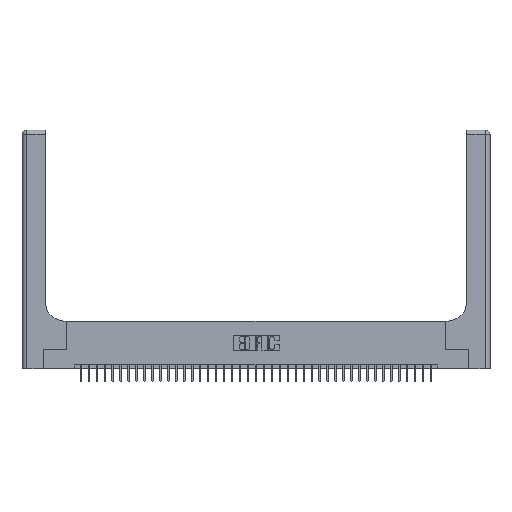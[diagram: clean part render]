
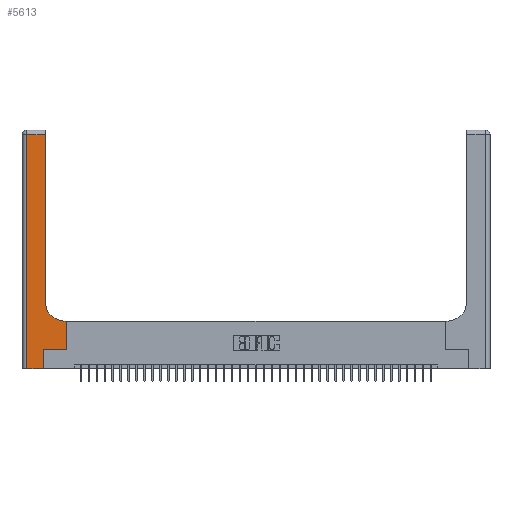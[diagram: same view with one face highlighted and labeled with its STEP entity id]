
A CAD part, top view. The second image highlights one B-rep face of the part: STEP entity #5613.
In plain terms, the highlighted planar face has unit normal (0, 0, 1).
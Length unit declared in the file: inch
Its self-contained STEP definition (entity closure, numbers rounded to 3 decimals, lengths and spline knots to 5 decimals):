
#130 = CARTESIAN_POINT ( 'NONE',  ( 0.06, 3., 0.37 ) ) ;
#830 = VECTOR ( 'NONE', #20768, 39.37008 ) ;
#1373 = CARTESIAN_POINT ( 'NONE',  ( 0.5415, 0.85, 0.37 ) ) ;
#3284 = DIRECTION ( 'NONE',  ( 0., -1., 0. ) ) ;
#3754 = CARTESIAN_POINT ( 'NONE',  ( 0.5585, 0.6, 0.37 ) ) ;
#3790 = VERTEX_POINT ( 'NONE', #15621 ) ;
#4520 = DIRECTION ( 'NONE',  ( 1., 0., 0. ) ) ;
#4714 = LINE ( 'NONE', #38202, #35749 ) ;
#4879 = LINE ( 'NONE', #14296, #12200 ) ;
#4936 = DIRECTION ( 'NONE',  ( 0., 1., 0. ) ) ;
#4947 = VECTOR ( 'NONE', #11902, 39.37008 ) ;
#5030 = ORIENTED_EDGE ( 'NONE', *, *, #28999, .T. ) ;
#5613 = ADVANCED_FACE ( 'NONE', ( #12121 ), #33946, .F. ) ;
#6167 = DIRECTION ( 'NONE',  ( -1., 0., 0. ) ) ;
#6580 = VERTEX_POINT ( 'NONE', #35375 ) ;
#6622 = DIRECTION ( 'NONE',  ( 1., 0., 0. ) ) ;
#7062 = EDGE_CURVE ( 'NONE', #3790, #25156, #9646, .T. ) ;
#7198 = LINE ( 'NONE', #130, #15441 ) ;
#9646 = LINE ( 'NONE', #15824, #23162 ) ;
#10445 = EDGE_CURVE ( 'NONE', #6580, #27169, #28688, .T. ) ;
#11052 = CARTESIAN_POINT ( 'NONE',  ( 0., 2.94, 0.37 ) ) ;
#11204 = ORIENTED_EDGE ( 'NONE', *, *, #7062, .T. ) ;
#11902 = DIRECTION ( 'NONE',  ( 0., 1., 0. ) ) ;
#12121 = FACE_OUTER_BOUND ( 'NONE', #28138, .T. ) ;
#12200 = VECTOR ( 'NONE', #4936, 39.37008 ) ;
#12298 = CARTESIAN_POINT ( 'NONE',  ( 0., 3., 0.37 ) ) ;
#13057 = DIRECTION ( 'NONE',  ( -1., 0., 0. ) ) ;
#13212 = LINE ( 'NONE', #14846, #4947 ) ;
#14142 = DIRECTION ( 'NONE',  ( -1., 0., 0. ) ) ;
#14296 = CARTESIAN_POINT ( 'NONE',  ( 0.5585, 0.25, 0.37 ) ) ;
#14688 = LINE ( 'NONE', #28485, #38421 ) ;
#14846 = CARTESIAN_POINT ( 'NONE',  ( 0.2915, 3., 0.37 ) ) ;
#15441 = VECTOR ( 'NONE', #3284, 39.37008 ) ;
#15621 = CARTESIAN_POINT ( 'NONE',  ( 0.06, 0., 0.37 ) ) ;
#15824 = CARTESIAN_POINT ( 'NONE',  ( 0., 0., 0.37 ) ) ;
#16118 = CARTESIAN_POINT ( 'NONE',  ( 0.5415, 0.6, 0.37 ) ) ;
#16372 = EDGE_CURVE ( 'NONE', #21794, #37944, #4879, .T. ) ;
#16645 = VERTEX_POINT ( 'NONE', #27847 ) ;
#16713 = VERTEX_POINT ( 'NONE', #21866 ) ;
#17464 = CIRCLE ( 'NONE', #35033, 0.25 ) ;
#17623 = CARTESIAN_POINT ( 'NONE',  ( 0.269, 0.25, 0.37 ) ) ;
#17897 = ORIENTED_EDGE ( 'NONE', *, *, #31254, .T. ) ;
#18410 = AXIS2_PLACEMENT_3D ( 'NONE', #12298, #24723, #6167 ) ;
#18676 = VERTEX_POINT ( 'NONE', #16118 ) ;
#19835 = EDGE_CURVE ( 'NONE', #16713, #6580, #13212, .T. ) ;
#20459 = VECTOR ( 'NONE', #14142, 39.37008 ) ;
#20768 = DIRECTION ( 'NONE',  ( 1., 0., 0. ) ) ;
#20869 = ORIENTED_EDGE ( 'NONE', *, *, #10445, .T. ) ;
#21530 = CARTESIAN_POINT ( 'NONE',  ( 0.5585, 0.25, 0.37 ) ) ;
#21794 = VERTEX_POINT ( 'NONE', #21530 ) ;
#21866 = CARTESIAN_POINT ( 'NONE',  ( 0.2915, 0.85, 0.37 ) ) ;
#22688 = CARTESIAN_POINT ( 'NONE',  ( 0.06, 2.94, 0.37 ) ) ;
#22755 = DIRECTION ( 'NONE',  ( 0., 1., 0. ) ) ;
#23087 = DIRECTION ( 'NONE',  ( 0., 0., -1. ) ) ;
#23162 = VECTOR ( 'NONE', #6622, 39.37008 ) ;
#24457 = CARTESIAN_POINT ( 'NONE',  ( 0.269, 0., 0.37 ) ) ;
#24723 = DIRECTION ( 'NONE',  ( 0., 0., -1. ) ) ;
#25156 = VERTEX_POINT ( 'NONE', #24457 ) ;
#25208 = ORIENTED_EDGE ( 'NONE', *, *, #19835, .T. ) ;
#25587 = LINE ( 'NONE', #17623, #830 ) ;
#27169 = VERTEX_POINT ( 'NONE', #22688 ) ;
#27688 = EDGE_CURVE ( 'NONE', #37944, #18676, #14688, .T. ) ;
#27847 = CARTESIAN_POINT ( 'NONE',  ( 0.269, 0.25, 0.37 ) ) ;
#28138 = EDGE_LOOP ( 'NONE', ( #25208, #20869, #17897, #11204, #39095, #33312, #31360, #33047, #5030 ) ) ;
#28485 = CARTESIAN_POINT ( 'NONE',  ( 0.2915, 0.6, 0.37 ) ) ;
#28688 = LINE ( 'NONE', #11052, #20459 ) ;
#28999 = EDGE_CURVE ( 'NONE', #18676, #16713, #17464, .T. ) ;
#31254 = EDGE_CURVE ( 'NONE', #27169, #3790, #7198, .T. ) ;
#31360 = ORIENTED_EDGE ( 'NONE', *, *, #16372, .T. ) ;
#31620 = EDGE_CURVE ( 'NONE', #16645, #21794, #25587, .T. ) ;
#31981 = EDGE_CURVE ( 'NONE', #25156, #16645, #4714, .T. ) ;
#33047 = ORIENTED_EDGE ( 'NONE', *, *, #27688, .T. ) ;
#33312 = ORIENTED_EDGE ( 'NONE', *, *, #31620, .T. ) ;
#33946 = PLANE ( 'NONE',  #18410 ) ;
#35033 = AXIS2_PLACEMENT_3D ( 'NONE', #1373, #23087, #4520 ) ;
#35375 = CARTESIAN_POINT ( 'NONE',  ( 0.2915, 2.94, 0.37 ) ) ;
#35749 = VECTOR ( 'NONE', #22755, 39.37008 ) ;
#37944 = VERTEX_POINT ( 'NONE', #3754 ) ;
#38202 = CARTESIAN_POINT ( 'NONE',  ( 0.269, 0., 0.37 ) ) ;
#38421 = VECTOR ( 'NONE', #13057, 39.37008 ) ;
#39095 = ORIENTED_EDGE ( 'NONE', *, *, #31981, .T. ) ;
